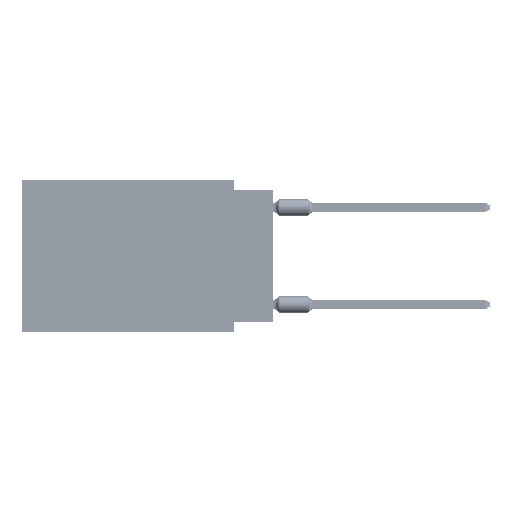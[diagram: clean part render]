
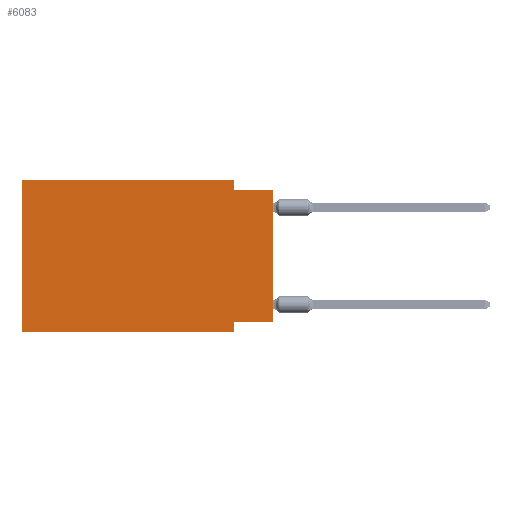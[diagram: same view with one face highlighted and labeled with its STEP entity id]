
A CAD part, left-side view. The second image highlights one B-rep face of the part: STEP entity #6083.
In plain terms, the highlighted planar face has unit normal (-1, 0, 0).
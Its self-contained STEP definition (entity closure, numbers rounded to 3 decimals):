
#481 = ORIENTED_EDGE ( 'NONE', *, *, #23310, .T. ) ;
#810 = VECTOR ( 'NONE', #5308, 1000. ) ;
#2834 = VERTEX_POINT ( 'NONE', #41710 ) ;
#3355 = ORIENTED_EDGE ( 'NONE', *, *, #18284, .F. ) ;
#5308 = DIRECTION ( 'NONE',  ( 0., -1., 0. ) ) ;
#5778 = DIRECTION ( 'NONE',  ( 0., 0., -1. ) ) ;
#6042 = CARTESIAN_POINT ( 'NONE',  ( 0., 0., -0.635 ) ) ;
#6083 = ADVANCED_FACE ( 'NONE', ( #32932 ), #39111, .F. ) ;
#6560 = VECTOR ( 'NONE', #67713, 1000. ) ;
#6737 = LINE ( 'NONE', #18701, #17184 ) ;
#6757 = VECTOR ( 'NONE', #71771, 1000. ) ;
#6971 = ORIENTED_EDGE ( 'NONE', *, *, #53315, .F. ) ;
#7765 = ORIENTED_EDGE ( 'NONE', *, *, #58129, .T. ) ;
#9846 = LINE ( 'NONE', #37469, #10357 ) ;
#10357 = VECTOR ( 'NONE', #14579, 1000. ) ;
#10807 = VERTEX_POINT ( 'NONE', #28040 ) ;
#11213 = CARTESIAN_POINT ( 'NONE',  ( 0., 2.54, 0. ) ) ;
#13351 = VECTOR ( 'NONE', #71175, 1000. ) ;
#13523 = CARTESIAN_POINT ( 'NONE',  ( 0., 0., -0.635 ) ) ;
#14579 = DIRECTION ( 'NONE',  ( 0., 0., 1. ) ) ;
#17184 = VECTOR ( 'NONE', #35077, 1000. ) ;
#18284 = EDGE_CURVE ( 'NONE', #62733, #44352, #67073, .T. ) ;
#18701 = CARTESIAN_POINT ( 'NONE',  ( 0., 16.383, 0. ) ) ;
#21309 = CARTESIAN_POINT ( 'NONE',  ( 0., 16.383, -9.906 ) ) ;
#21422 = EDGE_CURVE ( 'NONE', #38044, #10807, #49240, .T. ) ;
#22751 = DIRECTION ( 'NONE',  ( 1., 0., 0. ) ) ;
#23310 = EDGE_CURVE ( 'NONE', #68697, #44352, #9846, .T. ) ;
#24404 = CARTESIAN_POINT ( 'NONE',  ( 0., 2.54, -9.271 ) ) ;
#24652 = CARTESIAN_POINT ( 'NONE',  ( 0., 16.383, -9.906 ) ) ;
#25295 = EDGE_LOOP ( 'NONE', ( #481, #3355, #58142, #66213, #54106, #7765, #6971, #37301 ) ) ;
#28040 = CARTESIAN_POINT ( 'NONE',  ( 0., 16.383, 0. ) ) ;
#32932 = FACE_OUTER_BOUND ( 'NONE', #25295, .T. ) ;
#33471 = CARTESIAN_POINT ( 'NONE',  ( 0., 0., -9.271 ) ) ;
#35077 = DIRECTION ( 'NONE',  ( 0., -1., 0. ) ) ;
#37301 = ORIENTED_EDGE ( 'NONE', *, *, #65855, .F. ) ;
#37469 = CARTESIAN_POINT ( 'NONE',  ( 0., 0., 0. ) ) ;
#38044 = VERTEX_POINT ( 'NONE', #21309 ) ;
#39111 = PLANE ( 'NONE',  #56794 ) ;
#41710 = CARTESIAN_POINT ( 'NONE',  ( 0., 2.54, 0. ) ) ;
#42094 = VERTEX_POINT ( 'NONE', #24404 ) ;
#44352 = VERTEX_POINT ( 'NONE', #13523 ) ;
#44488 = CARTESIAN_POINT ( 'NONE',  ( 0., 0., -9.271 ) ) ;
#47735 = CARTESIAN_POINT ( 'NONE',  ( 0., 2.54, -0.635 ) ) ;
#48165 = VECTOR ( 'NONE', #5778, 1000. ) ;
#48995 = LINE ( 'NONE', #11213, #13351 ) ;
#49240 = LINE ( 'NONE', #60872, #6757 ) ;
#49983 = CARTESIAN_POINT ( 'NONE',  ( 0., 16.383, 0. ) ) ;
#51188 = DIRECTION ( 'NONE',  ( 0., -1., 0. ) ) ;
#53309 = EDGE_CURVE ( 'NONE', #2834, #62733, #48995, .T. ) ;
#53315 = EDGE_CURVE ( 'NONE', #42094, #65371, #60994, .T. ) ;
#54106 = ORIENTED_EDGE ( 'NONE', *, *, #21422, .F. ) ;
#55447 = CARTESIAN_POINT ( 'NONE',  ( 0., 2.54, -9.906 ) ) ;
#55530 = CARTESIAN_POINT ( 'NONE',  ( 0., 2.54, -9.906 ) ) ;
#56084 = LINE ( 'NONE', #44488, #6560 ) ;
#56794 = AXIS2_PLACEMENT_3D ( 'NONE', #49983, #22751, #61972 ) ;
#58129 = EDGE_CURVE ( 'NONE', #38044, #65371, #62446, .T. ) ;
#58142 = ORIENTED_EDGE ( 'NONE', *, *, #53309, .F. ) ;
#60872 = CARTESIAN_POINT ( 'NONE',  ( 0., 16.383, 0. ) ) ;
#60994 = LINE ( 'NONE', #55530, #48165 ) ;
#61972 = DIRECTION ( 'NONE',  ( 0., 0., -1. ) ) ;
#62446 = LINE ( 'NONE', #24652, #70987 ) ;
#62733 = VERTEX_POINT ( 'NONE', #47735 ) ;
#65371 = VERTEX_POINT ( 'NONE', #55447 ) ;
#65855 = EDGE_CURVE ( 'NONE', #68697, #42094, #56084, .T. ) ;
#66213 = ORIENTED_EDGE ( 'NONE', *, *, #67850, .F. ) ;
#67073 = LINE ( 'NONE', #6042, #810 ) ;
#67713 = DIRECTION ( 'NONE',  ( 0., 1., 0. ) ) ;
#67850 = EDGE_CURVE ( 'NONE', #10807, #2834, #6737, .T. ) ;
#68697 = VERTEX_POINT ( 'NONE', #33471 ) ;
#70987 = VECTOR ( 'NONE', #51188, 1000. ) ;
#71175 = DIRECTION ( 'NONE',  ( 0., 0., -1. ) ) ;
#71771 = DIRECTION ( 'NONE',  ( 0., 0., 1. ) ) ;
